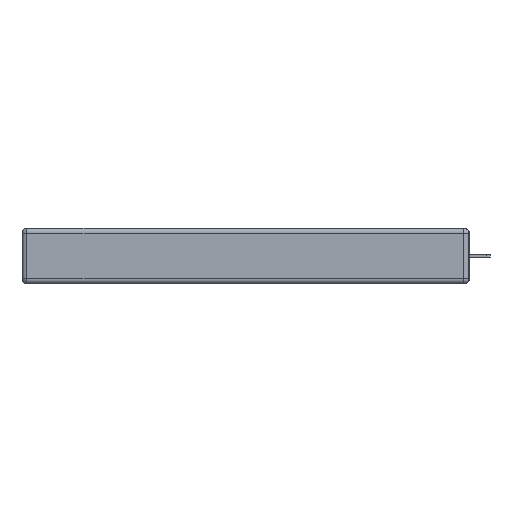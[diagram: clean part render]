
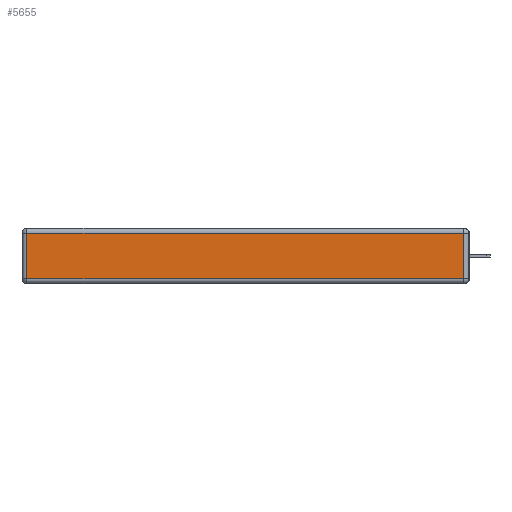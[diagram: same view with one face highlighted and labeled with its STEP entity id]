
A CAD part, left-side view. The second image highlights one B-rep face of the part: STEP entity #5655.
In plain terms, the highlighted planar face has unit normal (-1, 0, 0).
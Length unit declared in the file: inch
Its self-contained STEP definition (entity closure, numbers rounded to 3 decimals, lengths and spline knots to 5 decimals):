
#1488 = CARTESIAN_POINT ( 'NONE',  ( 0., 0.03, -0.03 ) ) ;
#2166 = LINE ( 'NONE', #22137, #11303 ) ;
#2245 = PLANE ( 'NONE',  #5667 ) ;
#2987 = VECTOR ( 'NONE', #4913, 39.37008 ) ;
#2992 = CARTESIAN_POINT ( 'NONE',  ( 0., 2.72, -0.343 ) ) ;
#3084 = CARTESIAN_POINT ( 'NONE',  ( 0., 0., -0.313 ) ) ;
#3663 = CARTESIAN_POINT ( 'NONE',  ( 0., 2.72, -0.313 ) ) ;
#4044 = DIRECTION ( 'NONE',  ( 0., 0., 1. ) ) ;
#4436 = EDGE_CURVE ( 'NONE', #11839, #11121, #19603, .T. ) ;
#4913 = DIRECTION ( 'NONE',  ( 0., -1., 0. ) ) ;
#5655 = ADVANCED_FACE ( 'NONE', ( #7434 ), #2245, .T. ) ;
#5667 = AXIS2_PLACEMENT_3D ( 'NONE', #11332, #14942, #4044 ) ;
#6021 = CARTESIAN_POINT ( 'NONE',  ( 0., 0.03, -0.343 ) ) ;
#6505 = CARTESIAN_POINT ( 'NONE',  ( 0., 2.72, -0.03 ) ) ;
#7120 = CARTESIAN_POINT ( 'NONE',  ( 0., 0.03, -0.313 ) ) ;
#7434 = FACE_OUTER_BOUND ( 'NONE', #7766, .T. ) ;
#7766 = EDGE_LOOP ( 'NONE', ( #11598, #8396, #13814, #21353 ) ) ;
#8085 = VERTEX_POINT ( 'NONE', #6505 ) ;
#8396 = ORIENTED_EDGE ( 'NONE', *, *, #4436, .T. ) ;
#8397 = LINE ( 'NONE', #3084, #2987 ) ;
#8552 = EDGE_CURVE ( 'NONE', #11121, #8085, #2166, .T. ) ;
#10070 = VECTOR ( 'NONE', #22227, 39.37008 ) ;
#11121 = VERTEX_POINT ( 'NONE', #1488 ) ;
#11303 = VECTOR ( 'NONE', #20338, 39.37008 ) ;
#11332 = CARTESIAN_POINT ( 'NONE',  ( 0., 0., -0.343 ) ) ;
#11598 = ORIENTED_EDGE ( 'NONE', *, *, #15409, .T. ) ;
#11839 = VERTEX_POINT ( 'NONE', #7120 ) ;
#13060 = VERTEX_POINT ( 'NONE', #3663 ) ;
#13814 = ORIENTED_EDGE ( 'NONE', *, *, #8552, .T. ) ;
#14942 = DIRECTION ( 'NONE',  ( -1., 0., 0. ) ) ;
#15409 = EDGE_CURVE ( 'NONE', #13060, #11839, #8397, .T. ) ;
#15785 = EDGE_CURVE ( 'NONE', #8085, #13060, #22709, .T. ) ;
#17953 = VECTOR ( 'NONE', #22776, 39.37008 ) ;
#19603 = LINE ( 'NONE', #6021, #10070 ) ;
#20338 = DIRECTION ( 'NONE',  ( 0., 1., 0. ) ) ;
#21353 = ORIENTED_EDGE ( 'NONE', *, *, #15785, .T. ) ;
#22137 = CARTESIAN_POINT ( 'NONE',  ( 0., 2.75, -0.03 ) ) ;
#22227 = DIRECTION ( 'NONE',  ( 0., 0., 1. ) ) ;
#22709 = LINE ( 'NONE', #2992, #17953 ) ;
#22776 = DIRECTION ( 'NONE',  ( 0., 0., -1. ) ) ;
